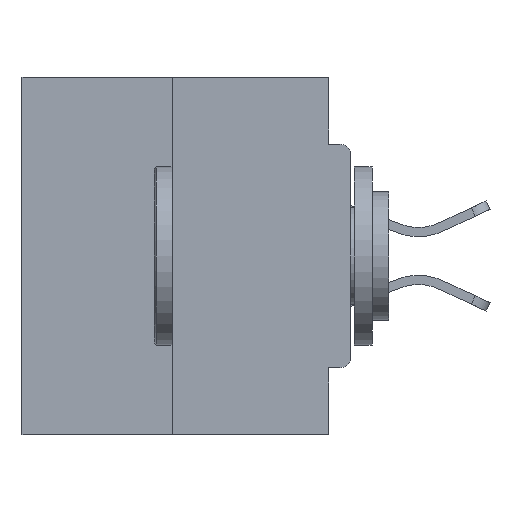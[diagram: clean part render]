
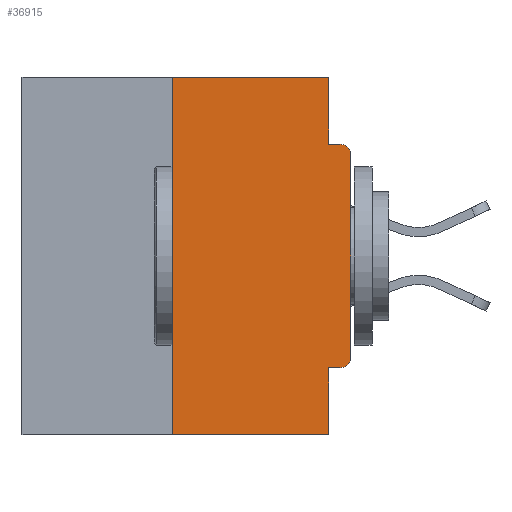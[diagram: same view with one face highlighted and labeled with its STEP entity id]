
A CAD part, left-side view. The second image highlights one B-rep face of the part: STEP entity #36915.
In plain terms, the highlighted planar face has unit normal (-1, 0, 0).
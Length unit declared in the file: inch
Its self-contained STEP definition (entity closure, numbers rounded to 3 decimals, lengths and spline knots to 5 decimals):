
#14 = ORIENTED_EDGE ( 'NONE', *, *, #16763, .T. ) ;
#171 = ORIENTED_EDGE ( 'NONE', *, *, #35961, .F. ) ;
#392 = LINE ( 'NONE', #3705, #28922 ) ;
#682 = LINE ( 'NONE', #29920, #9055 ) ;
#702 = ORIENTED_EDGE ( 'NONE', *, *, #10376, .F. ) ;
#975 = DIRECTION ( 'NONE',  ( 0., -1., 0. ) ) ;
#1735 = CARTESIAN_POINT ( 'NONE',  ( 0., 0.015, -0.1085 ) ) ;
#1906 = CARTESIAN_POINT ( 'NONE',  ( 0., 0.25, -0.5 ) ) ;
#2041 = CIRCLE ( 'NONE', #32479, 0.015 ) ;
#3167 = ORIENTED_EDGE ( 'NONE', *, *, #35114, .T. ) ;
#3543 = VECTOR ( 'NONE', #37879, 39.37008 ) ;
#3705 = CARTESIAN_POINT ( 'NONE',  ( 0., 0., -0.0935 ) ) ;
#3993 = VERTEX_POINT ( 'NONE', #24996 ) ;
#4722 = DIRECTION ( 'NONE',  ( 0., 0., -1. ) ) ;
#5268 = LINE ( 'NONE', #16285, #18636 ) ;
#5827 = VERTEX_POINT ( 'NONE', #7996 ) ;
#6113 = CARTESIAN_POINT ( 'NONE',  ( 0., 0.46, 0. ) ) ;
#6164 = LINE ( 'NONE', #9835, #27308 ) ;
#6501 = VERTEX_POINT ( 'NONE', #33223 ) ;
#6702 = VERTEX_POINT ( 'NONE', #28367 ) ;
#7791 = DIRECTION ( 'NONE',  ( -1., 0., 0. ) ) ;
#7857 = EDGE_CURVE ( 'NONE', #13171, #5827, #34291, .T. ) ;
#7922 = CARTESIAN_POINT ( 'NONE',  ( 0., 0.015, -0.0935 ) ) ;
#7996 = CARTESIAN_POINT ( 'NONE',  ( 0., 0.25, 0. ) ) ;
#8968 = DIRECTION ( 'NONE',  ( 0., 0., -1. ) ) ;
#8982 = VERTEX_POINT ( 'NONE', #7922 ) ;
#9055 = VECTOR ( 'NONE', #9514, 39.37008 ) ;
#9514 = DIRECTION ( 'NONE',  ( 0., -1., 0. ) ) ;
#9655 = AXIS2_PLACEMENT_3D ( 'NONE', #1735, #7791, #4722 ) ;
#9835 = CARTESIAN_POINT ( 'NONE',  ( 0., 0.031, 0. ) ) ;
#10376 = EDGE_CURVE ( 'NONE', #11702, #27384, #13837, .T. ) ;
#11622 = PLANE ( 'NONE',  #29654 ) ;
#11670 = VECTOR ( 'NONE', #22659, 39.37008 ) ;
#11702 = VERTEX_POINT ( 'NONE', #17757 ) ;
#12332 = CARTESIAN_POINT ( 'NONE',  ( 0., 0.031, -0.4065 ) ) ;
#12577 = ORIENTED_EDGE ( 'NONE', *, *, #33434, .F. ) ;
#12746 = DIRECTION ( 'NONE',  ( 0., 0., -1. ) ) ;
#13058 = ORIENTED_EDGE ( 'NONE', *, *, #37895, .F. ) ;
#13171 = VERTEX_POINT ( 'NONE', #1906 ) ;
#13289 = CIRCLE ( 'NONE', #9655, 0.015 ) ;
#13837 = LINE ( 'NONE', #18913, #26226 ) ;
#14879 = CARTESIAN_POINT ( 'NONE',  ( 0., 0.015, -0.3915 ) ) ;
#16285 = CARTESIAN_POINT ( 'NONE',  ( 0., 0.46, 0. ) ) ;
#16763 = EDGE_CURVE ( 'NONE', #13171, #6702, #682, .T. ) ;
#17705 = DIRECTION ( 'NONE',  ( 0., 0., -1. ) ) ;
#17757 = CARTESIAN_POINT ( 'NONE',  ( 0., 0.015, -0.4065 ) ) ;
#17858 = CARTESIAN_POINT ( 'NONE',  ( 0., 0.031, 0. ) ) ;
#17943 = DIRECTION ( 'NONE',  ( 1., 0., 0. ) ) ;
#18636 = VECTOR ( 'NONE', #19231, 39.37008 ) ;
#18913 = CARTESIAN_POINT ( 'NONE',  ( 0., 0., -0.4065 ) ) ;
#19231 = DIRECTION ( 'NONE',  ( 0., -1., 0. ) ) ;
#20688 = EDGE_CURVE ( 'NONE', #11702, #6501, #2041, .T. ) ;
#21135 = EDGE_CURVE ( 'NONE', #27384, #6702, #24986, .T. ) ;
#21743 = VERTEX_POINT ( 'NONE', #17858 ) ;
#22220 = DIRECTION ( 'NONE',  ( 0., 1., 0. ) ) ;
#22659 = DIRECTION ( 'NONE',  ( 0., 0., -1. ) ) ;
#22692 = FACE_OUTER_BOUND ( 'NONE', #34394, .T. ) ;
#23290 = LINE ( 'NONE', #26040, #3543 ) ;
#24986 = LINE ( 'NONE', #28307, #11670 ) ;
#24996 = CARTESIAN_POINT ( 'NONE',  ( 0., 0.031, -0.0935 ) ) ;
#25071 = ORIENTED_EDGE ( 'NONE', *, *, #20688, .T. ) ;
#26040 = CARTESIAN_POINT ( 'NONE',  ( 0., 0., 0. ) ) ;
#26226 = VECTOR ( 'NONE', #22220, 39.37008 ) ;
#27123 = VERTEX_POINT ( 'NONE', #37268 ) ;
#27308 = VECTOR ( 'NONE', #12746, 39.37008 ) ;
#27384 = VERTEX_POINT ( 'NONE', #12332 ) ;
#27757 = ORIENTED_EDGE ( 'NONE', *, *, #7857, .F. ) ;
#28071 = ORIENTED_EDGE ( 'NONE', *, *, #21135, .F. ) ;
#28262 = VECTOR ( 'NONE', #28387, 39.37008 ) ;
#28307 = CARTESIAN_POINT ( 'NONE',  ( 0., 0.031, -0.5 ) ) ;
#28367 = CARTESIAN_POINT ( 'NONE',  ( 0., 0.031, -0.5 ) ) ;
#28387 = DIRECTION ( 'NONE',  ( 0., 0., 1. ) ) ;
#28922 = VECTOR ( 'NONE', #975, 39.37008 ) ;
#29654 = AXIS2_PLACEMENT_3D ( 'NONE', #6113, #17943, #8968 ) ;
#29920 = CARTESIAN_POINT ( 'NONE',  ( 0., 0.46, -0.5 ) ) ;
#32479 = AXIS2_PLACEMENT_3D ( 'NONE', #14879, #35312, #17705 ) ;
#33223 = CARTESIAN_POINT ( 'NONE',  ( 0., 0., -0.3915 ) ) ;
#33434 = EDGE_CURVE ( 'NONE', #3993, #8982, #392, .T. ) ;
#33442 = EDGE_CURVE ( 'NONE', #27123, #8982, #13289, .T. ) ;
#34291 = LINE ( 'NONE', #36896, #28262 ) ;
#34394 = EDGE_LOOP ( 'NONE', ( #171, #27757, #14, #28071, #702, #25071, #3167, #37781, #12577, #13058 ) ) ;
#35114 = EDGE_CURVE ( 'NONE', #6501, #27123, #23290, .T. ) ;
#35312 = DIRECTION ( 'NONE',  ( -1., 0., 0. ) ) ;
#35961 = EDGE_CURVE ( 'NONE', #5827, #21743, #5268, .T. ) ;
#36896 = CARTESIAN_POINT ( 'NONE',  ( 0., 0.25, 0. ) ) ;
#36915 = ADVANCED_FACE ( 'NONE', ( #22692 ), #11622, .F. ) ;
#37268 = CARTESIAN_POINT ( 'NONE',  ( 0., 0., -0.1085 ) ) ;
#37781 = ORIENTED_EDGE ( 'NONE', *, *, #33442, .T. ) ;
#37879 = DIRECTION ( 'NONE',  ( 0., 0., 1. ) ) ;
#37895 = EDGE_CURVE ( 'NONE', #21743, #3993, #6164, .T. ) ;
